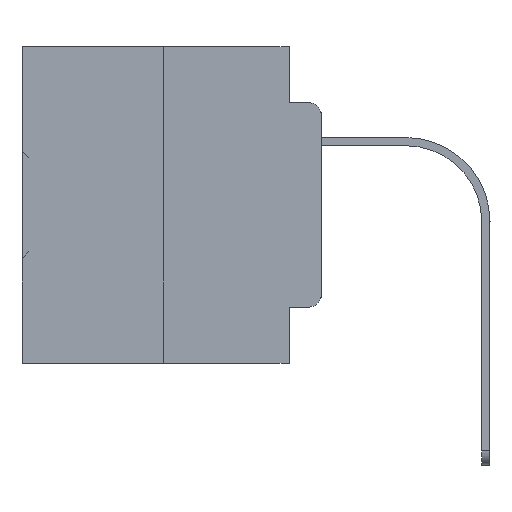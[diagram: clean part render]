
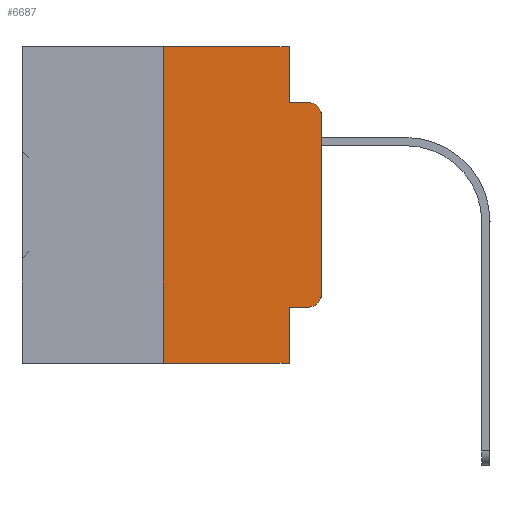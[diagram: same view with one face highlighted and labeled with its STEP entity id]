
A CAD part, left-side view. The second image highlights one B-rep face of the part: STEP entity #6687.
In plain terms, the highlighted planar face has unit normal (-1, 0, 0).
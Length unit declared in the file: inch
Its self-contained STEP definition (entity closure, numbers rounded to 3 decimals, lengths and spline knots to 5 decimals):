
#115 = ORIENTED_EDGE ( 'NONE', *, *, #22063, .T. ) ;
#240 = VERTEX_POINT ( 'NONE', #5092 ) ;
#1295 = EDGE_CURVE ( 'NONE', #3822, #5553, #12473, .T. ) ;
#1435 = FACE_OUTER_BOUND ( 'NONE', #26047, .T. ) ;
#2952 = EDGE_CURVE ( 'NONE', #20360, #26010, #33717, .T. ) ;
#3004 = ORIENTED_EDGE ( 'NONE', *, *, #4650, .F. ) ;
#3085 = CARTESIAN_POINT ( 'NONE',  ( 0., 0.473, -0.5 ) ) ;
#3510 = DIRECTION ( 'NONE',  ( 0., 0., -1. ) ) ;
#3822 = VERTEX_POINT ( 'NONE', #12952 ) ;
#4452 = CARTESIAN_POINT ( 'NONE',  ( 0., 0.473, 0. ) ) ;
#4650 = EDGE_CURVE ( 'NONE', #36513, #17081, #14317, .T. ) ;
#4894 = DIRECTION ( 'NONE',  ( 0., 0., 1. ) ) ;
#5092 = CARTESIAN_POINT ( 'NONE',  ( 0., 0.051, 0. ) ) ;
#5553 = VERTEX_POINT ( 'NONE', #29592 ) ;
#6440 = EDGE_CURVE ( 'NONE', #5553, #16094, #15608, .T. ) ;
#6687 = ADVANCED_FACE ( 'NONE', ( #1435 ), #12926, .F. ) ;
#7024 = CARTESIAN_POINT ( 'NONE',  ( 0., 0.051, 0. ) ) ;
#7347 = VECTOR ( 'NONE', #12307, 39.37008 ) ;
#7418 = VERTEX_POINT ( 'NONE', #35210 ) ;
#7763 = VERTEX_POINT ( 'NONE', #12010 ) ;
#9028 = LINE ( 'NONE', #26168, #27549 ) ;
#9052 = CARTESIAN_POINT ( 'NONE',  ( 0., 0.25, -0.5 ) ) ;
#9156 = VECTOR ( 'NONE', #33943, 39.37008 ) ;
#10227 = LINE ( 'NONE', #7024, #7347 ) ;
#11069 = EDGE_CURVE ( 'NONE', #7418, #16094, #9028, .T. ) ;
#11622 = ORIENTED_EDGE ( 'NONE', *, *, #2952, .F. ) ;
#11761 = VECTOR ( 'NONE', #25237, 39.37008 ) ;
#11996 = CARTESIAN_POINT ( 'NONE',  ( 0., 0.051, -0.4115 ) ) ;
#12003 = DIRECTION ( 'NONE',  ( -1., 0., 0. ) ) ;
#12010 = CARTESIAN_POINT ( 'NONE',  ( 0., 0.02, -0.4115 ) ) ;
#12307 = DIRECTION ( 'NONE',  ( 0., 0., -1. ) ) ;
#12455 = DIRECTION ( 'NONE',  ( -1., 0., 0. ) ) ;
#12473 = LINE ( 'NONE', #32819, #17639 ) ;
#12897 = VECTOR ( 'NONE', #15432, 39.37008 ) ;
#12926 = PLANE ( 'NONE',  #15986 ) ;
#12952 = CARTESIAN_POINT ( 'NONE',  ( 0., 0., -0.3915 ) ) ;
#13112 = DIRECTION ( 'NONE',  ( 1., 0., 0. ) ) ;
#13615 = ORIENTED_EDGE ( 'NONE', *, *, #26086, .F. ) ;
#14065 = ORIENTED_EDGE ( 'NONE', *, *, #14697, .F. ) ;
#14317 = LINE ( 'NONE', #36550, #11761 ) ;
#14697 = EDGE_CURVE ( 'NONE', #26010, #240, #21782, .T. ) ;
#14944 = VECTOR ( 'NONE', #20465, 39.37008 ) ;
#15185 = CARTESIAN_POINT ( 'NONE',  ( 0., 0.051, -0.5 ) ) ;
#15432 = DIRECTION ( 'NONE',  ( 0., -1., 0. ) ) ;
#15608 = CIRCLE ( 'NONE', #33610, 0.02 ) ;
#15684 = CARTESIAN_POINT ( 'NONE',  ( 0., 0.02, -0.3915 ) ) ;
#15986 = AXIS2_PLACEMENT_3D ( 'NONE', #4452, #13112, #36101 ) ;
#16094 = VERTEX_POINT ( 'NONE', #37047 ) ;
#17081 = VERTEX_POINT ( 'NONE', #15185 ) ;
#17639 = VECTOR ( 'NONE', #26414, 39.37008 ) ;
#17931 = ORIENTED_EDGE ( 'NONE', *, *, #33086, .T. ) ;
#18328 = DIRECTION ( 'NONE',  ( 0., 0., -1. ) ) ;
#20360 = VERTEX_POINT ( 'NONE', #9052 ) ;
#20465 = DIRECTION ( 'NONE',  ( 0., -1., 0. ) ) ;
#21566 = CARTESIAN_POINT ( 'NONE',  ( 0., 0.25, 0. ) ) ;
#21782 = LINE ( 'NONE', #29716, #12897 ) ;
#22063 = EDGE_CURVE ( 'NONE', #20360, #17081, #31917, .T. ) ;
#22484 = LINE ( 'NONE', #26329, #9156 ) ;
#22660 = ORIENTED_EDGE ( 'NONE', *, *, #30848, .T. ) ;
#23317 = CARTESIAN_POINT ( 'NONE',  ( 0., 0.02, -0.1085 ) ) ;
#25237 = DIRECTION ( 'NONE',  ( 0., 0., -1. ) ) ;
#26010 = VERTEX_POINT ( 'NONE', #21566 ) ;
#26047 = EDGE_LOOP ( 'NONE', ( #29682, #35532, #29638, #13615, #14065, #11622, #115, #3004, #17931, #22660 ) ) ;
#26086 = EDGE_CURVE ( 'NONE', #240, #7418, #10227, .T. ) ;
#26168 = CARTESIAN_POINT ( 'NONE',  ( 0., 0.051, -0.0885 ) ) ;
#26329 = CARTESIAN_POINT ( 'NONE',  ( 0., 0.051, -0.4115 ) ) ;
#26414 = DIRECTION ( 'NONE',  ( 0., 0., 1. ) ) ;
#27549 = VECTOR ( 'NONE', #29184, 39.37008 ) ;
#27804 = AXIS2_PLACEMENT_3D ( 'NONE', #15684, #12455, #18328 ) ;
#28069 = CARTESIAN_POINT ( 'NONE',  ( 0., 0.25, 0. ) ) ;
#28425 = CIRCLE ( 'NONE', #27804, 0.02 ) ;
#29184 = DIRECTION ( 'NONE',  ( 0., -1., 0. ) ) ;
#29592 = CARTESIAN_POINT ( 'NONE',  ( 0., 0., -0.1085 ) ) ;
#29638 = ORIENTED_EDGE ( 'NONE', *, *, #11069, .F. ) ;
#29682 = ORIENTED_EDGE ( 'NONE', *, *, #1295, .T. ) ;
#29716 = CARTESIAN_POINT ( 'NONE',  ( 0., 0.473, 0. ) ) ;
#30848 = EDGE_CURVE ( 'NONE', #7763, #3822, #28425, .T. ) ;
#31566 = VECTOR ( 'NONE', #4894, 39.37008 ) ;
#31917 = LINE ( 'NONE', #3085, #14944 ) ;
#32819 = CARTESIAN_POINT ( 'NONE',  ( 0., 0., 0. ) ) ;
#33086 = EDGE_CURVE ( 'NONE', #36513, #7763, #22484, .T. ) ;
#33610 = AXIS2_PLACEMENT_3D ( 'NONE', #23317, #12003, #3510 ) ;
#33717 = LINE ( 'NONE', #28069, #31566 ) ;
#33943 = DIRECTION ( 'NONE',  ( 0., -1., 0. ) ) ;
#35210 = CARTESIAN_POINT ( 'NONE',  ( 0., 0.051, -0.0885 ) ) ;
#35532 = ORIENTED_EDGE ( 'NONE', *, *, #6440, .T. ) ;
#36101 = DIRECTION ( 'NONE',  ( 0., 0., -1. ) ) ;
#36513 = VERTEX_POINT ( 'NONE', #11996 ) ;
#36550 = CARTESIAN_POINT ( 'NONE',  ( 0., 0.051, 0. ) ) ;
#37047 = CARTESIAN_POINT ( 'NONE',  ( 0., 0.02, -0.0885 ) ) ;
